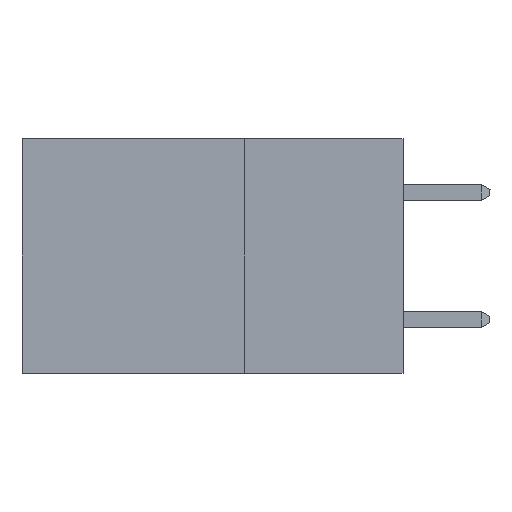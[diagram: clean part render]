
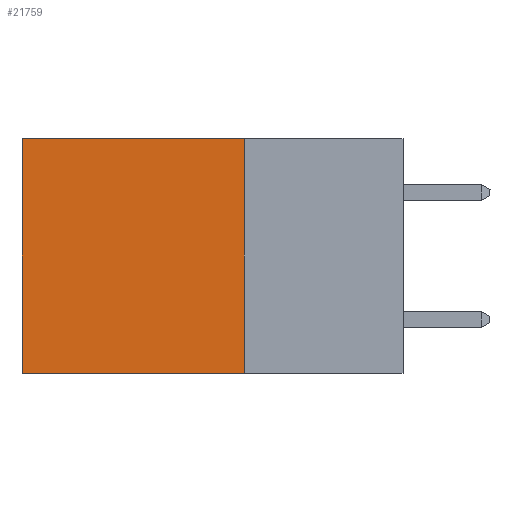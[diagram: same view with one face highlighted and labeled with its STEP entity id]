
A CAD part, left-side view. The second image highlights one B-rep face of the part: STEP entity #21759.
In plain terms, the highlighted planar face has unit normal (-1, 0, 0).
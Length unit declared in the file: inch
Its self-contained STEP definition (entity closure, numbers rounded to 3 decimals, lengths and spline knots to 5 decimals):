
#19 = EDGE_CURVE ( 'NONE', #3265, #29340, #29514, .T. ) ;
#33 = LINE ( 'NONE', #7496, #6366 ) ;
#237 = VERTEX_POINT ( 'NONE', #20354 ) ;
#3265 = VERTEX_POINT ( 'NONE', #32276 ) ;
#3858 = ORIENTED_EDGE ( 'NONE', *, *, #19, .T. ) ;
#6366 = VECTOR ( 'NONE', #26269, 39.37008 ) ;
#7496 = CARTESIAN_POINT ( 'NONE',  ( 0.2875, 0.25, -0.37 ) ) ;
#8846 = DIRECTION ( 'NONE',  ( 0., 1., 0. ) ) ;
#9128 = ORIENTED_EDGE ( 'NONE', *, *, #22971, .F. ) ;
#9797 = VERTEX_POINT ( 'NONE', #22066 ) ;
#10407 = DIRECTION ( 'NONE',  ( 0., 0., -1. ) ) ;
#11879 = VECTOR ( 'NONE', #20432, 39.37008 ) ;
#13013 = VECTOR ( 'NONE', #21736, 39.37008 ) ;
#13566 = EDGE_CURVE ( 'NONE', #29340, #237, #20103, .T. ) ;
#15689 = CARTESIAN_POINT ( 'NONE',  ( 0.2875, 0.25, 0. ) ) ;
#16142 = FACE_OUTER_BOUND ( 'NONE', #18589, .T. ) ;
#18377 = PLANE ( 'NONE',  #20502 ) ;
#18589 = EDGE_LOOP ( 'NONE', ( #32274, #9128, #31033, #3858 ) ) ;
#20103 = LINE ( 'NONE', #29722, #13013 ) ;
#20354 = CARTESIAN_POINT ( 'NONE',  ( 0.2875, 0.6, -0.37 ) ) ;
#20432 = DIRECTION ( 'NONE',  ( 0., 0., -1. ) ) ;
#20502 = AXIS2_PLACEMENT_3D ( 'NONE', #15689, #26452, #10407 ) ;
#21736 = DIRECTION ( 'NONE',  ( 0., 0., -1. ) ) ;
#21759 = ADVANCED_FACE ( 'NONE', ( #16142 ), #18377, .F. ) ;
#22066 = CARTESIAN_POINT ( 'NONE',  ( 0.2875, 0.25, -0.37 ) ) ;
#22357 = VECTOR ( 'NONE', #8846, 39.37008 ) ;
#22971 = EDGE_CURVE ( 'NONE', #9797, #237, #33, .T. ) ;
#24956 = CARTESIAN_POINT ( 'NONE',  ( 0.2875, 0.25, 0. ) ) ;
#26269 = DIRECTION ( 'NONE',  ( 0., 1., 0. ) ) ;
#26452 = DIRECTION ( 'NONE',  ( 1., 0., 0. ) ) ;
#26967 = LINE ( 'NONE', #28389, #11879 ) ;
#28389 = CARTESIAN_POINT ( 'NONE',  ( 0.2875, 0.25, 0. ) ) ;
#28729 = EDGE_CURVE ( 'NONE', #3265, #9797, #26967, .T. ) ;
#29340 = VERTEX_POINT ( 'NONE', #31049 ) ;
#29514 = LINE ( 'NONE', #24956, #22357 ) ;
#29722 = CARTESIAN_POINT ( 'NONE',  ( 0.2875, 0.6, 0. ) ) ;
#31033 = ORIENTED_EDGE ( 'NONE', *, *, #28729, .F. ) ;
#31049 = CARTESIAN_POINT ( 'NONE',  ( 0.2875, 0.6, 0. ) ) ;
#32274 = ORIENTED_EDGE ( 'NONE', *, *, #13566, .T. ) ;
#32276 = CARTESIAN_POINT ( 'NONE',  ( 0.2875, 0.25, 0. ) ) ;
